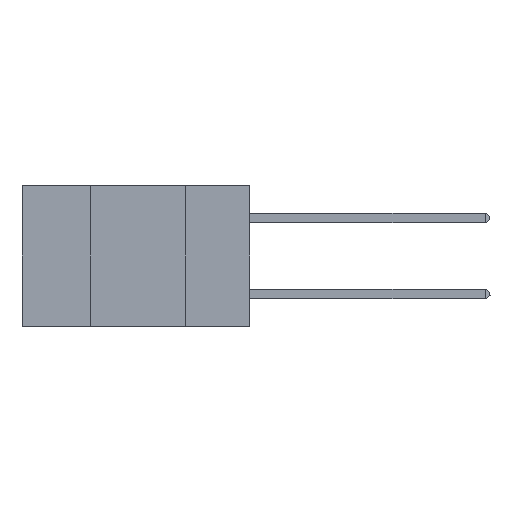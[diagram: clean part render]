
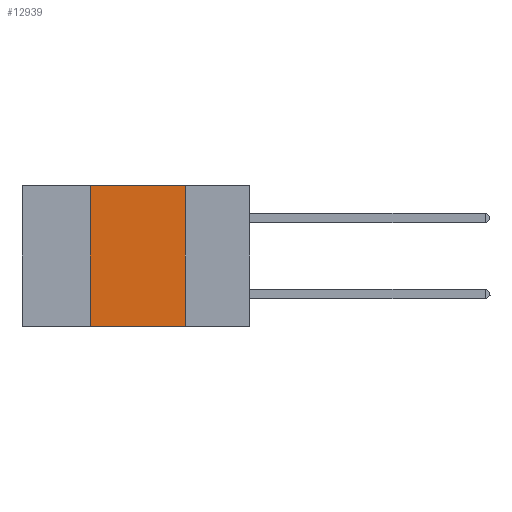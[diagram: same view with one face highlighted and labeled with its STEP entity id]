
A CAD part, left-side view. The second image highlights one B-rep face of the part: STEP entity #12939.
In plain terms, the highlighted planar face has unit normal (-1, 0, 0).
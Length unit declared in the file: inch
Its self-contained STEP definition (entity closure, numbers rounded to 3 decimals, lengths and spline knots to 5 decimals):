
#181 = DIRECTION ( 'NONE',  ( 1., 0., 0. ) ) ;
#399 = LINE ( 'NONE', #20263, #16465 ) ;
#1407 = CARTESIAN_POINT ( 'NONE',  ( 0., 0.42, -0.37 ) ) ;
#2116 = CARTESIAN_POINT ( 'NONE',  ( 0., 0.17, 0. ) ) ;
#2137 = FACE_OUTER_BOUND ( 'NONE', #6531, .T. ) ;
#2143 = VECTOR ( 'NONE', #18222, 39.37008 ) ;
#2424 = DIRECTION ( 'NONE',  ( 0., 0., 1. ) ) ;
#3777 = PLANE ( 'NONE',  #4161 ) ;
#3961 = VERTEX_POINT ( 'NONE', #1407 ) ;
#4161 = AXIS2_PLACEMENT_3D ( 'NONE', #19341, #181, #12402 ) ;
#4535 = VECTOR ( 'NONE', #19583, 39.37008 ) ;
#6531 = EDGE_LOOP ( 'NONE', ( #17005, #15393, #11325, #14619 ) ) ;
#7140 = EDGE_CURVE ( 'NONE', #11708, #12941, #399, .T. ) ;
#10219 = VERTEX_POINT ( 'NONE', #18761 ) ;
#11325 = ORIENTED_EDGE ( 'NONE', *, *, #18380, .F. ) ;
#11708 = VERTEX_POINT ( 'NONE', #13750 ) ;
#12402 = DIRECTION ( 'NONE',  ( 0., 0., -1. ) ) ;
#12939 = ADVANCED_FACE ( 'NONE', ( #2137 ), #3777, .F. ) ;
#12941 = VERTEX_POINT ( 'NONE', #14125 ) ;
#13066 = LINE ( 'NONE', #14716, #2143 ) ;
#13750 = CARTESIAN_POINT ( 'NONE',  ( 0., 0.42, 0. ) ) ;
#13795 = LINE ( 'NONE', #2116, #4535 ) ;
#13953 = VECTOR ( 'NONE', #2424, 39.37008 ) ;
#14125 = CARTESIAN_POINT ( 'NONE',  ( 0., 0.17, 0. ) ) ;
#14437 = CARTESIAN_POINT ( 'NONE',  ( 0., 0.42, 0. ) ) ;
#14619 = ORIENTED_EDGE ( 'NONE', *, *, #20360, .T. ) ;
#14716 = CARTESIAN_POINT ( 'NONE',  ( 0., 0.6, -0.37 ) ) ;
#15393 = ORIENTED_EDGE ( 'NONE', *, *, #7140, .F. ) ;
#16465 = VECTOR ( 'NONE', #22007, 39.37008 ) ;
#17005 = ORIENTED_EDGE ( 'NONE', *, *, #21568, .F. ) ;
#18222 = DIRECTION ( 'NONE',  ( 0., -1., 0. ) ) ;
#18380 = EDGE_CURVE ( 'NONE', #3961, #11708, #22196, .T. ) ;
#18761 = CARTESIAN_POINT ( 'NONE',  ( 0., 0.17, -0.37 ) ) ;
#19341 = CARTESIAN_POINT ( 'NONE',  ( 0., 0.6, 0. ) ) ;
#19583 = DIRECTION ( 'NONE',  ( 0., 0., -1. ) ) ;
#20263 = CARTESIAN_POINT ( 'NONE',  ( 0., 0.6, 0. ) ) ;
#20360 = EDGE_CURVE ( 'NONE', #3961, #10219, #13066, .T. ) ;
#21568 = EDGE_CURVE ( 'NONE', #12941, #10219, #13795, .T. ) ;
#22007 = DIRECTION ( 'NONE',  ( 0., -1., 0. ) ) ;
#22196 = LINE ( 'NONE', #14437, #13953 ) ;
